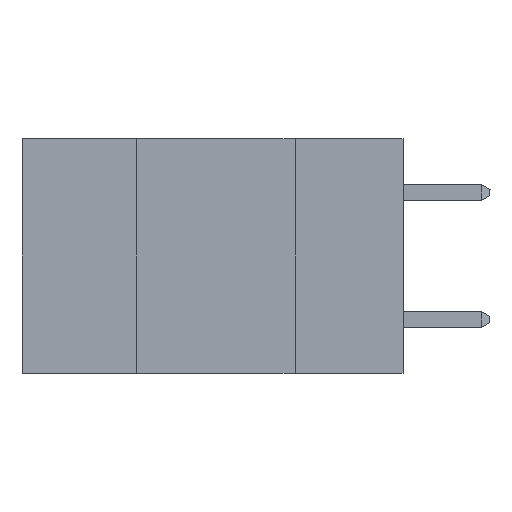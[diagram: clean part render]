
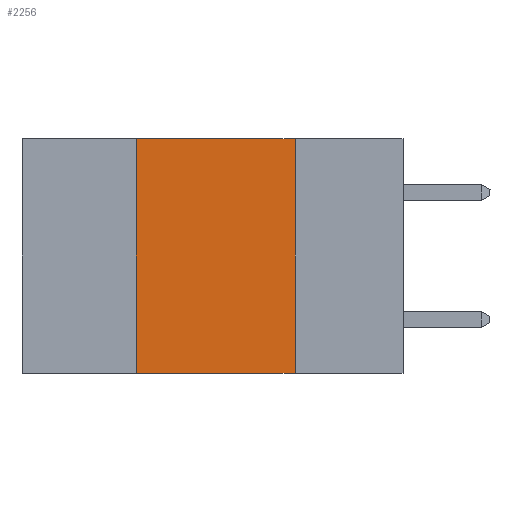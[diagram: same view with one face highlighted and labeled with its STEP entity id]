
A CAD part, left-side view. The second image highlights one B-rep face of the part: STEP entity #2256.
In plain terms, the highlighted planar face has unit normal (-1, 0, 0).
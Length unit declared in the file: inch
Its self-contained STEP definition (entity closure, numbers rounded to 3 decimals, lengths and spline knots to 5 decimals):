
#309 = CARTESIAN_POINT ( 'NONE',  ( 0., 0.42, 0. ) ) ;
#596 = VERTEX_POINT ( 'NONE', #7868 ) ;
#1246 = VECTOR ( 'NONE', #4719, 39.37008 ) ;
#1366 = EDGE_CURVE ( 'NONE', #14184, #596, #7616, .T. ) ;
#1490 = LINE ( 'NONE', #13912, #4078 ) ;
#1610 = CARTESIAN_POINT ( 'NONE',  ( 0., 0.42, 0. ) ) ;
#2256 = ADVANCED_FACE ( 'NONE', ( #7065 ), #12172, .F. ) ;
#2636 = CARTESIAN_POINT ( 'NONE',  ( 0., 0.17, 0. ) ) ;
#3464 = CARTESIAN_POINT ( 'NONE',  ( 0., 0.6, 0. ) ) ;
#3493 = LINE ( 'NONE', #2636, #1246 ) ;
#3501 = DIRECTION ( 'NONE',  ( 1., 0., 0. ) ) ;
#3635 = ORIENTED_EDGE ( 'NONE', *, *, #5820, .F. ) ;
#3931 = EDGE_CURVE ( 'NONE', #596, #4316, #3493, .T. ) ;
#4078 = VECTOR ( 'NONE', #5112, 39.37008 ) ;
#4316 = VERTEX_POINT ( 'NONE', #10169 ) ;
#4719 = DIRECTION ( 'NONE',  ( 0., 0., -1. ) ) ;
#4754 = DIRECTION ( 'NONE',  ( 0., 0., -1. ) ) ;
#5112 = DIRECTION ( 'NONE',  ( 0., -1., 0. ) ) ;
#5169 = ORIENTED_EDGE ( 'NONE', *, *, #3931, .F. ) ;
#5820 = EDGE_CURVE ( 'NONE', #11957, #14184, #13759, .T. ) ;
#5950 = EDGE_LOOP ( 'NONE', ( #5169, #9058, #3635, #7336 ) ) ;
#6716 = CARTESIAN_POINT ( 'NONE',  ( 0., 0.42, -0.37 ) ) ;
#7048 = EDGE_CURVE ( 'NONE', #11957, #4316, #1490, .T. ) ;
#7065 = FACE_OUTER_BOUND ( 'NONE', #5950, .T. ) ;
#7336 = ORIENTED_EDGE ( 'NONE', *, *, #7048, .T. ) ;
#7390 = AXIS2_PLACEMENT_3D ( 'NONE', #10237, #3501, #4754 ) ;
#7616 = LINE ( 'NONE', #3464, #9862 ) ;
#7868 = CARTESIAN_POINT ( 'NONE',  ( 0., 0.17, 0. ) ) ;
#8063 = VECTOR ( 'NONE', #9361, 39.37008 ) ;
#9058 = ORIENTED_EDGE ( 'NONE', *, *, #1366, .F. ) ;
#9361 = DIRECTION ( 'NONE',  ( 0., 0., 1. ) ) ;
#9862 = VECTOR ( 'NONE', #12278, 39.37008 ) ;
#10169 = CARTESIAN_POINT ( 'NONE',  ( 0., 0.17, -0.37 ) ) ;
#10237 = CARTESIAN_POINT ( 'NONE',  ( 0., 0.6, 0. ) ) ;
#11957 = VERTEX_POINT ( 'NONE', #6716 ) ;
#12172 = PLANE ( 'NONE',  #7390 ) ;
#12278 = DIRECTION ( 'NONE',  ( 0., -1., 0. ) ) ;
#13759 = LINE ( 'NONE', #1610, #8063 ) ;
#13912 = CARTESIAN_POINT ( 'NONE',  ( 0., 0.6, -0.37 ) ) ;
#14184 = VERTEX_POINT ( 'NONE', #309 ) ;
